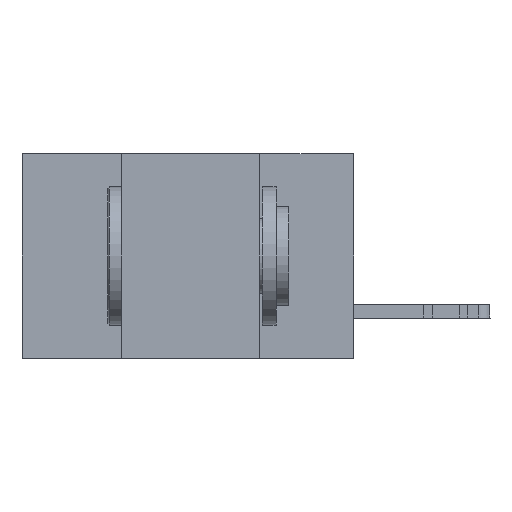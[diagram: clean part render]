
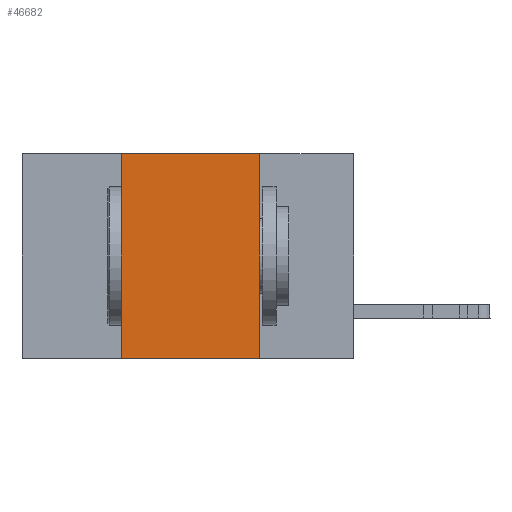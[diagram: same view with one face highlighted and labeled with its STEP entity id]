
A CAD part, left-side view. The second image highlights one B-rep face of the part: STEP entity #46682.
In plain terms, the highlighted planar face has unit normal (-1, 0, 0).
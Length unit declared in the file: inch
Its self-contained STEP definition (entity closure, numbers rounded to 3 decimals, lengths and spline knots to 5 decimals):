
#135 = CARTESIAN_POINT ( 'NONE',  ( 0., 0.17, 0. ) ) ;
#4261 = VERTEX_POINT ( 'NONE', #42194 ) ;
#7368 = VERTEX_POINT ( 'NONE', #44093 ) ;
#8999 = LINE ( 'NONE', #28930, #30774 ) ;
#9630 = ORIENTED_EDGE ( 'NONE', *, *, #29191, .F. ) ;
#9762 = DIRECTION ( 'NONE',  ( 0., 0., 1. ) ) ;
#12198 = CARTESIAN_POINT ( 'NONE',  ( 0., 0.6, 0. ) ) ;
#13568 = DIRECTION ( 'NONE',  ( 1., 0., 0. ) ) ;
#15484 = DIRECTION ( 'NONE',  ( 0., -1., 0. ) ) ;
#15812 = VERTEX_POINT ( 'NONE', #28240 ) ;
#16420 = CARTESIAN_POINT ( 'NONE',  ( 0., 0.17, -0.37 ) ) ;
#16889 = EDGE_CURVE ( 'NONE', #15812, #30240, #40486, .T. ) ;
#20336 = VECTOR ( 'NONE', #42414, 39.37008 ) ;
#21854 = DIRECTION ( 'NONE',  ( 0., -1., 0. ) ) ;
#23037 = VECTOR ( 'NONE', #21854, 39.37008 ) ;
#23464 = ORIENTED_EDGE ( 'NONE', *, *, #16889, .F. ) ;
#25833 = EDGE_CURVE ( 'NONE', #7368, #30240, #36983, .T. ) ;
#26878 = CARTESIAN_POINT ( 'NONE',  ( 0., 0.6, -0.37 ) ) ;
#28240 = CARTESIAN_POINT ( 'NONE',  ( 0., 0.17, 0. ) ) ;
#28930 = CARTESIAN_POINT ( 'NONE',  ( 0., 0.42, 0. ) ) ;
#29164 = CARTESIAN_POINT ( 'NONE',  ( 0., 0.6, 0. ) ) ;
#29191 = EDGE_CURVE ( 'NONE', #4261, #15812, #41372, .T. ) ;
#30240 = VERTEX_POINT ( 'NONE', #16420 ) ;
#30594 = EDGE_LOOP ( 'NONE', ( #23464, #9630, #37203, #46761 ) ) ;
#30774 = VECTOR ( 'NONE', #9762, 39.37008 ) ;
#32484 = DIRECTION ( 'NONE',  ( 0., 0., -1. ) ) ;
#36983 = LINE ( 'NONE', #26878, #45917 ) ;
#37203 = ORIENTED_EDGE ( 'NONE', *, *, #41699, .F. ) ;
#37779 = FACE_OUTER_BOUND ( 'NONE', #30594, .T. ) ;
#40486 = LINE ( 'NONE', #135, #20336 ) ;
#40664 = PLANE ( 'NONE',  #41439 ) ;
#41372 = LINE ( 'NONE', #29164, #23037 ) ;
#41439 = AXIS2_PLACEMENT_3D ( 'NONE', #12198, #13568, #32484 ) ;
#41699 = EDGE_CURVE ( 'NONE', #7368, #4261, #8999, .T. ) ;
#42194 = CARTESIAN_POINT ( 'NONE',  ( 0., 0.42, 0. ) ) ;
#42414 = DIRECTION ( 'NONE',  ( 0., 0., -1. ) ) ;
#44093 = CARTESIAN_POINT ( 'NONE',  ( 0., 0.42, -0.37 ) ) ;
#45917 = VECTOR ( 'NONE', #15484, 39.37008 ) ;
#46682 = ADVANCED_FACE ( 'NONE', ( #37779 ), #40664, .F. ) ;
#46761 = ORIENTED_EDGE ( 'NONE', *, *, #25833, .T. ) ;
